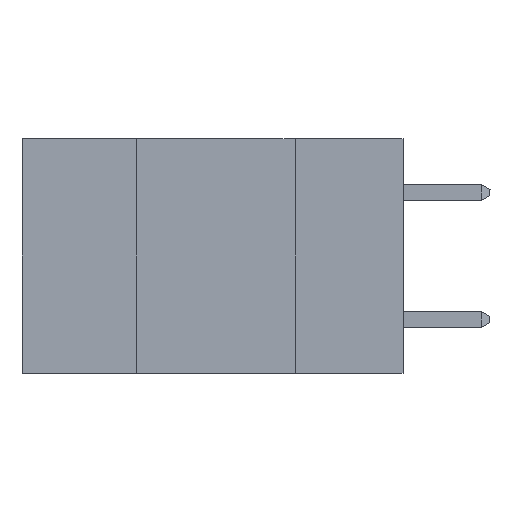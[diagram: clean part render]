
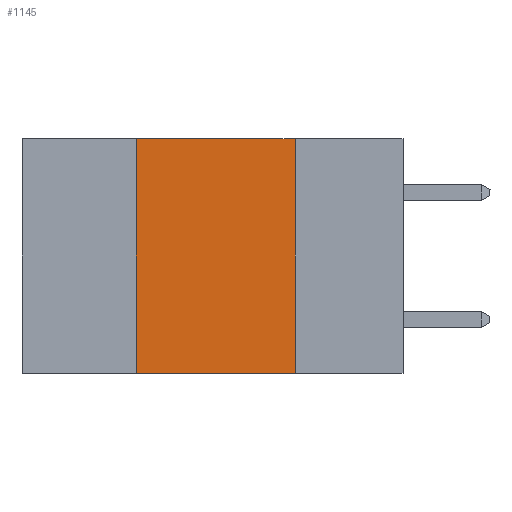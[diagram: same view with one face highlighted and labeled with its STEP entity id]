
A CAD part, left-side view. The second image highlights one B-rep face of the part: STEP entity #1145.
In plain terms, the highlighted planar face has unit normal (-1, 0, 0).
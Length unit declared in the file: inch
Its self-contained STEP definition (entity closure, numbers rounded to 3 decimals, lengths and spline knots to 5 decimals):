
#122 = EDGE_CURVE ( 'NONE', #2579, #16390, #15136, .T. ) ;
#1145 = ADVANCED_FACE ( 'NONE', ( #12346 ), #11518, .F. ) ;
#1280 = CARTESIAN_POINT ( 'NONE',  ( 0., 0.6, 0. ) ) ;
#1599 = DIRECTION ( 'NONE',  ( 1., 0., 0. ) ) ;
#1847 = EDGE_CURVE ( 'NONE', #20431, #6075, #16646, .T. ) ;
#2579 = VERTEX_POINT ( 'NONE', #18074 ) ;
#3947 = VECTOR ( 'NONE', #4767, 39.37008 ) ;
#3952 = ORIENTED_EDGE ( 'NONE', *, *, #16806, .T. ) ;
#4767 = DIRECTION ( 'NONE',  ( 0., 0., 1. ) ) ;
#4782 = VECTOR ( 'NONE', #7307, 39.37008 ) ;
#5657 = DIRECTION ( 'NONE',  ( 0., 0., -1. ) ) ;
#6075 = VERTEX_POINT ( 'NONE', #23624 ) ;
#6077 = VECTOR ( 'NONE', #5657, 39.37008 ) ;
#6338 = CARTESIAN_POINT ( 'NONE',  ( 0., 0.42, 0. ) ) ;
#6655 = EDGE_CURVE ( 'NONE', #16390, #20431, #10069, .T. ) ;
#7307 = DIRECTION ( 'NONE',  ( 0., -1., 0. ) ) ;
#10069 = LINE ( 'NONE', #1280, #4782 ) ;
#11446 = CARTESIAN_POINT ( 'NONE',  ( 0., 0.6, -0.37 ) ) ;
#11518 = PLANE ( 'NONE',  #17939 ) ;
#12346 = FACE_OUTER_BOUND ( 'NONE', #17014, .T. ) ;
#13289 = ORIENTED_EDGE ( 'NONE', *, *, #6655, .F. ) ;
#13511 = CARTESIAN_POINT ( 'NONE',  ( 0., 0.6, 0. ) ) ;
#15136 = LINE ( 'NONE', #18707, #3947 ) ;
#15502 = DIRECTION ( 'NONE',  ( 0., 0., -1. ) ) ;
#15547 = CARTESIAN_POINT ( 'NONE',  ( 0., 0.17, 0. ) ) ;
#15557 = CARTESIAN_POINT ( 'NONE',  ( 0., 0.17, 0. ) ) ;
#16390 = VERTEX_POINT ( 'NONE', #6338 ) ;
#16646 = LINE ( 'NONE', #15557, #6077 ) ;
#16806 = EDGE_CURVE ( 'NONE', #2579, #6075, #17684, .T. ) ;
#17014 = EDGE_LOOP ( 'NONE', ( #22019, #13289, #19229, #3952 ) ) ;
#17684 = LINE ( 'NONE', #11446, #23010 ) ;
#17939 = AXIS2_PLACEMENT_3D ( 'NONE', #13511, #1599, #15502 ) ;
#18074 = CARTESIAN_POINT ( 'NONE',  ( 0., 0.42, -0.37 ) ) ;
#18707 = CARTESIAN_POINT ( 'NONE',  ( 0., 0.42, 0. ) ) ;
#19229 = ORIENTED_EDGE ( 'NONE', *, *, #122, .F. ) ;
#20431 = VERTEX_POINT ( 'NONE', #15547 ) ;
#22019 = ORIENTED_EDGE ( 'NONE', *, *, #1847, .F. ) ;
#23010 = VECTOR ( 'NONE', #25418, 39.37008 ) ;
#23624 = CARTESIAN_POINT ( 'NONE',  ( 0., 0.17, -0.37 ) ) ;
#25418 = DIRECTION ( 'NONE',  ( 0., -1., 0. ) ) ;
